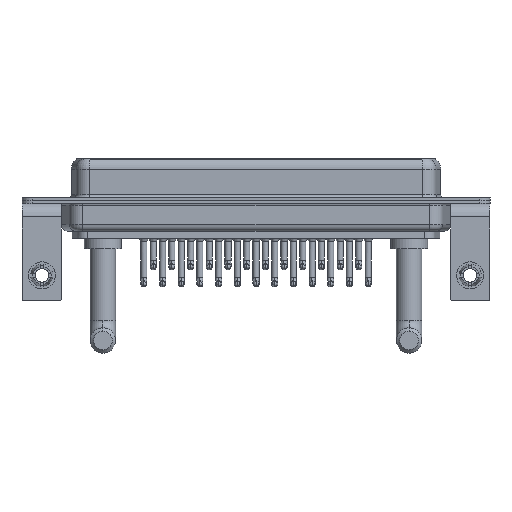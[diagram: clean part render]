
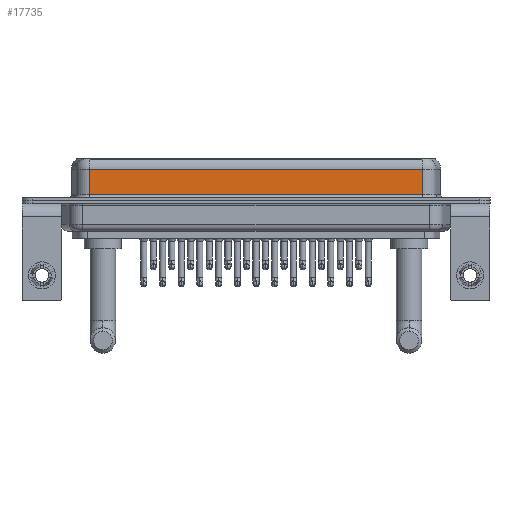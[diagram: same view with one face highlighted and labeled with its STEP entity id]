
A CAD part, front view. The second image highlights one B-rep face of the part: STEP entity #17735.
In plain terms, the highlighted planar face has unit normal (0, -1, 0).
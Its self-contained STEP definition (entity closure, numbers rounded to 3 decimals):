
#2472 = ORIENTED_EDGE ( 'NONE', *, *, #9470, .T. ) ;
#3142 = EDGE_CURVE ( 'NONE', #15209, #8476, #18251, .T. ) ;
#3645 = CARTESIAN_POINT ( 'NONE',  ( 7.038, -3.95, 6.4 ) ) ;
#3821 = VERTEX_POINT ( 'NONE', #8022 ) ;
#4069 = LINE ( 'NONE', #16480, #4169 ) ;
#4169 = VECTOR ( 'NONE', #12485, 1000. ) ;
#4922 = CARTESIAN_POINT ( 'NONE',  ( 56.462, -3.95, 0.9 ) ) ;
#5015 = AXIS2_PLACEMENT_3D ( 'NONE', #20332, #18373, #5575 ) ;
#5026 = FACE_OUTER_BOUND ( 'NONE', #8975, .T. ) ;
#5575 = DIRECTION ( 'NONE',  ( 0., 0., 1. ) ) ;
#5586 = DIRECTION ( 'NONE',  ( 0., 0., -1. ) ) ;
#6427 = EDGE_CURVE ( 'NONE', #3821, #6968, #18518, .T. ) ;
#6968 = VERTEX_POINT ( 'NONE', #20300 ) ;
#8022 = CARTESIAN_POINT ( 'NONE',  ( 7.038, -3.95, 4.65 ) ) ;
#8476 = VERTEX_POINT ( 'NONE', #14490 ) ;
#8742 = CARTESIAN_POINT ( 'NONE',  ( 56.462, -3.95, 4.65 ) ) ;
#8975 = EDGE_LOOP ( 'NONE', ( #26512, #2472, #16230, #26820 ) ) ;
#9470 = EDGE_CURVE ( 'NONE', #15209, #3821, #4069, .T. ) ;
#10080 = VECTOR ( 'NONE', #16588, 1000. ) ;
#11145 = DIRECTION ( 'NONE',  ( 1., 0., 0. ) ) ;
#12485 = DIRECTION ( 'NONE',  ( -1., 0., 0. ) ) ;
#13633 = VECTOR ( 'NONE', #5586, 1000. ) ;
#14125 = PLANE ( 'NONE',  #5015 ) ;
#14490 = CARTESIAN_POINT ( 'NONE',  ( 56.462, -3.95, 0.9 ) ) ;
#15209 = VERTEX_POINT ( 'NONE', #8742 ) ;
#15296 = VECTOR ( 'NONE', #11145, 1000. ) ;
#16230 = ORIENTED_EDGE ( 'NONE', *, *, #6427, .T. ) ;
#16480 = CARTESIAN_POINT ( 'NONE',  ( 56.462, -3.95, 4.65 ) ) ;
#16588 = DIRECTION ( 'NONE',  ( 0., 0., -1. ) ) ;
#17735 = ADVANCED_FACE ( 'NONE', ( #5026 ), #14125, .F. ) ;
#18251 = LINE ( 'NONE', #20210, #13633 ) ;
#18373 = DIRECTION ( 'NONE',  ( 0., 1., 0. ) ) ;
#18518 = LINE ( 'NONE', #3645, #10080 ) ;
#20210 = CARTESIAN_POINT ( 'NONE',  ( 56.462, -3.95, 6.4 ) ) ;
#20300 = CARTESIAN_POINT ( 'NONE',  ( 7.038, -3.95, 0.9 ) ) ;
#20332 = CARTESIAN_POINT ( 'NONE',  ( 56.462, -3.95, 6.4 ) ) ;
#20354 = EDGE_CURVE ( 'NONE', #6968, #8476, #21885, .T. ) ;
#21885 = LINE ( 'NONE', #4922, #15296 ) ;
#26512 = ORIENTED_EDGE ( 'NONE', *, *, #3142, .F. ) ;
#26820 = ORIENTED_EDGE ( 'NONE', *, *, #20354, .T. ) ;
